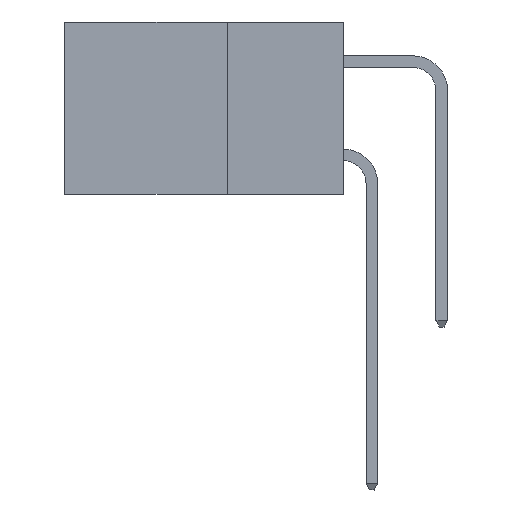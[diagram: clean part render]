
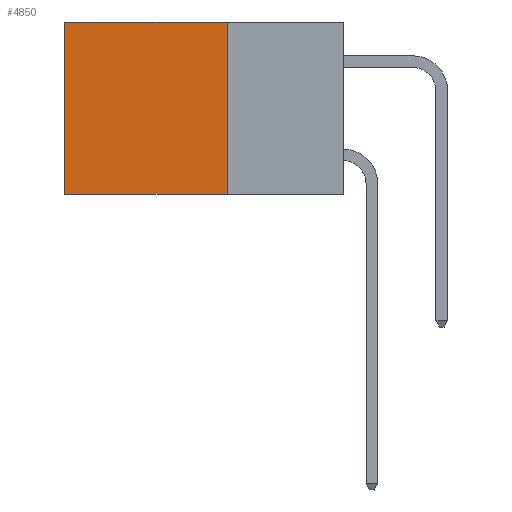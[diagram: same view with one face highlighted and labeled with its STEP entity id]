
A CAD part, left-side view. The second image highlights one B-rep face of the part: STEP entity #4850.
In plain terms, the highlighted planar face has unit normal (-1, 0, 0).
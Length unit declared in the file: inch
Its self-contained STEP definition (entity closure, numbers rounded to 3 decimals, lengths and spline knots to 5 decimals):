
#498 = CARTESIAN_POINT ( 'NONE',  ( 0.2615, 0.6, 0. ) ) ;
#1443 = FACE_OUTER_BOUND ( 'NONE', #10093, .T. ) ;
#1740 = VECTOR ( 'NONE', #10446, 39.37008 ) ;
#1745 = DIRECTION ( 'NONE',  ( 0., 0., -1. ) ) ;
#1987 = ORIENTED_EDGE ( 'NONE', *, *, #5267, .F. ) ;
#2243 = CARTESIAN_POINT ( 'NONE',  ( 0.2615, 0.25, 0. ) ) ;
#2387 = VERTEX_POINT ( 'NONE', #4263 ) ;
#2539 = ORIENTED_EDGE ( 'NONE', *, *, #9704, .T. ) ;
#2645 = VECTOR ( 'NONE', #1745, 39.37008 ) ;
#2846 = LINE ( 'NONE', #6142, #8051 ) ;
#3081 = DIRECTION ( 'NONE',  ( 1., 0., 0. ) ) ;
#3647 = VECTOR ( 'NONE', #8131, 39.37008 ) ;
#3726 = VERTEX_POINT ( 'NONE', #2243 ) ;
#4181 = VERTEX_POINT ( 'NONE', #4527 ) ;
#4186 = PLANE ( 'NONE',  #10376 ) ;
#4263 = CARTESIAN_POINT ( 'NONE',  ( 0.2615, 0.6, -0.37 ) ) ;
#4527 = CARTESIAN_POINT ( 'NONE',  ( 0.2615, 0.25, -0.37 ) ) ;
#4850 = ADVANCED_FACE ( 'NONE', ( #1443 ), #4186, .F. ) ;
#5019 = ORIENTED_EDGE ( 'NONE', *, *, #8598, .T. ) ;
#5267 = EDGE_CURVE ( 'NONE', #4181, #2387, #6644, .T. ) ;
#5592 = CARTESIAN_POINT ( 'NONE',  ( 0.2615, 0.25, -0.37 ) ) ;
#6142 = CARTESIAN_POINT ( 'NONE',  ( 0.2615, 0.25, 0. ) ) ;
#6484 = VERTEX_POINT ( 'NONE', #498 ) ;
#6633 = LINE ( 'NONE', #9251, #2645 ) ;
#6644 = LINE ( 'NONE', #5592, #3647 ) ;
#7536 = CARTESIAN_POINT ( 'NONE',  ( 0.2615, 0.25, -0.37 ) ) ;
#8051 = VECTOR ( 'NONE', #10368, 39.37008 ) ;
#8131 = DIRECTION ( 'NONE',  ( 0., 1., 0. ) ) ;
#8136 = CARTESIAN_POINT ( 'NONE',  ( 0.2615, 0.25, -0.37 ) ) ;
#8252 = DIRECTION ( 'NONE',  ( 0., 0., -1. ) ) ;
#8598 = EDGE_CURVE ( 'NONE', #3726, #6484, #2846, .T. ) ;
#9251 = CARTESIAN_POINT ( 'NONE',  ( 0.2615, 0.6, -0.37 ) ) ;
#9704 = EDGE_CURVE ( 'NONE', #6484, #2387, #6633, .T. ) ;
#9752 = ORIENTED_EDGE ( 'NONE', *, *, #10668, .F. ) ;
#9772 = LINE ( 'NONE', #8136, #1740 ) ;
#10093 = EDGE_LOOP ( 'NONE', ( #2539, #1987, #9752, #5019 ) ) ;
#10368 = DIRECTION ( 'NONE',  ( 0., 1., 0. ) ) ;
#10376 = AXIS2_PLACEMENT_3D ( 'NONE', #7536, #3081, #8252 ) ;
#10446 = DIRECTION ( 'NONE',  ( 0., 0., -1. ) ) ;
#10668 = EDGE_CURVE ( 'NONE', #3726, #4181, #9772, .T. ) ;
